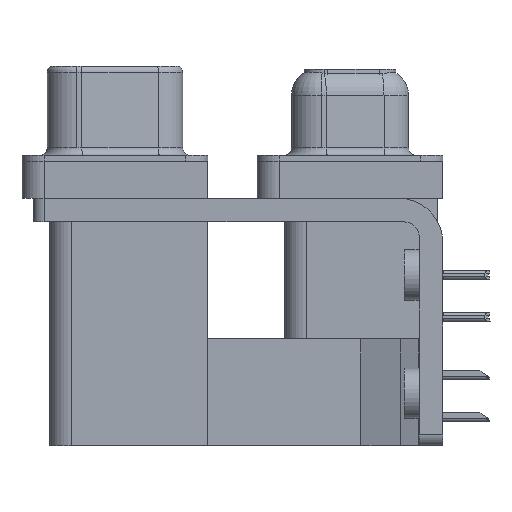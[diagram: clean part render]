
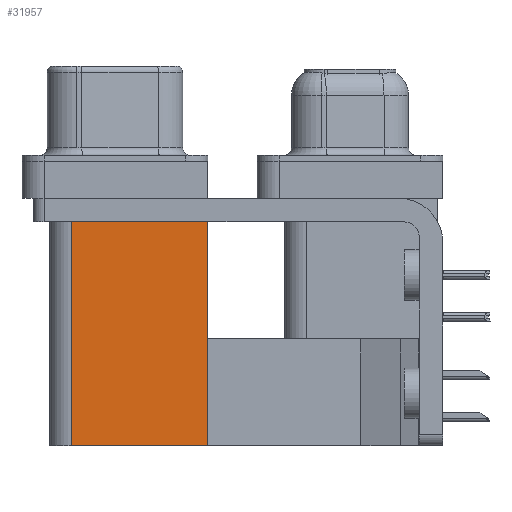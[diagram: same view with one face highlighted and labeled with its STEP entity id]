
A CAD part, left-side view. The second image highlights one B-rep face of the part: STEP entity #31957.
In plain terms, the highlighted planar face has unit normal (-1, 0, 0).
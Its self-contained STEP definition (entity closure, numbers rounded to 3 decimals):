
#129 = ORIENTED_EDGE ( 'NONE', *, *, #10291, .F. ) ;
#641 = ORIENTED_EDGE ( 'NONE', *, *, #6698, .T. ) ;
#3536 = AXIS2_PLACEMENT_3D ( 'NONE', #33203, #9471, #6075 ) ;
#6075 = DIRECTION ( 'NONE',  ( 0., 0., -1. ) ) ;
#6093 = VECTOR ( 'NONE', #33898, 1000. ) ;
#6302 = VERTEX_POINT ( 'NONE', #26300 ) ;
#6315 = VECTOR ( 'NONE', #6572, 1000. ) ;
#6572 = DIRECTION ( 'NONE',  ( 0., 1., 0. ) ) ;
#6698 = EDGE_CURVE ( 'NONE', #6302, #25083, #21607, .T. ) ;
#7025 = CARTESIAN_POINT ( 'NONE',  ( 3.79, 18.8, -19.2 ) ) ;
#7533 = LINE ( 'NONE', #32449, #19734 ) ;
#9360 = CARTESIAN_POINT ( 'NONE',  ( 3.79, 9.6, -2.5 ) ) ;
#9471 = DIRECTION ( 'NONE',  ( 1., 0., 0. ) ) ;
#10219 = ORIENTED_EDGE ( 'NONE', *, *, #29250, .F. ) ;
#10291 = EDGE_CURVE ( 'NONE', #32557, #35966, #7533, .T. ) ;
#11345 = ORIENTED_EDGE ( 'NONE', *, *, #31743, .T. ) ;
#15293 = FACE_OUTER_BOUND ( 'NONE', #33450, .T. ) ;
#15412 = VECTOR ( 'NONE', #19450, 1000. ) ;
#16040 = LINE ( 'NONE', #7025, #15412 ) ;
#16498 = CARTESIAN_POINT ( 'NONE',  ( 3.79, 18.8, -2.5 ) ) ;
#19450 = DIRECTION ( 'NONE',  ( 0., 0., 1. ) ) ;
#19734 = VECTOR ( 'NONE', #38870, 1000. ) ;
#21607 = LINE ( 'NONE', #9360, #6315 ) ;
#21613 = CARTESIAN_POINT ( 'NONE',  ( 3.79, 9.6, -19.2 ) ) ;
#25083 = VERTEX_POINT ( 'NONE', #16498 ) ;
#26300 = CARTESIAN_POINT ( 'NONE',  ( 3.79, 9.6, -2.5 ) ) ;
#27690 = CARTESIAN_POINT ( 'NONE',  ( 3.79, 9.6, -19.2 ) ) ;
#29250 = EDGE_CURVE ( 'NONE', #35966, #25083, #16040, .T. ) ;
#31743 = EDGE_CURVE ( 'NONE', #32557, #6302, #33702, .T. ) ;
#31957 = ADVANCED_FACE ( 'NONE', ( #15293 ), #33419, .F. ) ;
#32449 = CARTESIAN_POINT ( 'NONE',  ( 3.79, 9.6, -19.2 ) ) ;
#32557 = VERTEX_POINT ( 'NONE', #27690 ) ;
#32704 = CARTESIAN_POINT ( 'NONE',  ( 3.79, 18.8, -19.2 ) ) ;
#33203 = CARTESIAN_POINT ( 'NONE',  ( 3.79, 9.6, -19.2 ) ) ;
#33419 = PLANE ( 'NONE',  #3536 ) ;
#33450 = EDGE_LOOP ( 'NONE', ( #641, #10219, #129, #11345 ) ) ;
#33702 = LINE ( 'NONE', #21613, #6093 ) ;
#33898 = DIRECTION ( 'NONE',  ( 0., 0., 1. ) ) ;
#35966 = VERTEX_POINT ( 'NONE', #32704 ) ;
#38870 = DIRECTION ( 'NONE',  ( 0., 1., 0. ) ) ;
